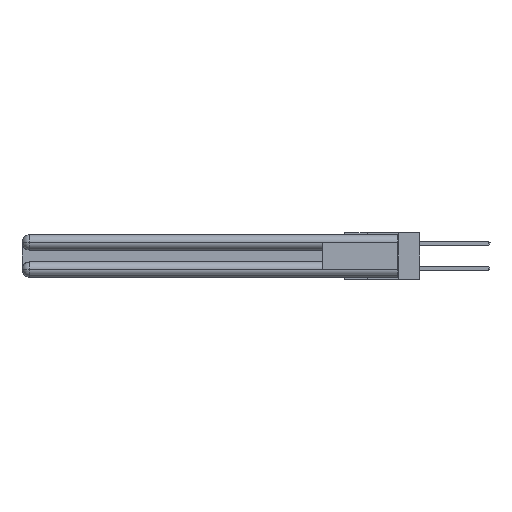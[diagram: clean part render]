
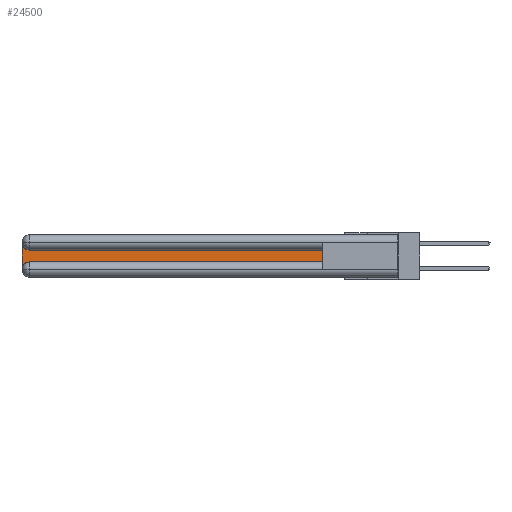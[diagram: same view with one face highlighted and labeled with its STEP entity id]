
A CAD part, left-side view. The second image highlights one B-rep face of the part: STEP entity #24500.
In plain terms, the highlighted planar face has unit normal (-1, 0, 0).
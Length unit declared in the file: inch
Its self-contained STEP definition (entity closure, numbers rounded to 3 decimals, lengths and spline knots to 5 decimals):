
#198 = DIRECTION ( 'NONE',  ( 0., 0., 1. ) ) ;
#234 = CARTESIAN_POINT ( 'NONE',  ( 0.075, 2.94, -0.0625 ) ) ;
#450 = ORIENTED_EDGE ( 'NONE', *, *, #9087, .T. ) ;
#917 = LINE ( 'NONE', #4924, #21539 ) ;
#2057 = VERTEX_POINT ( 'NONE', #13671 ) ;
#2864 = CARTESIAN_POINT ( 'NONE',  ( 0.075, 2.94, -0.2775 ) ) ;
#3566 = EDGE_CURVE ( 'NONE', #9020, #15563, #11306, .T. ) ;
#3692 = CARTESIAN_POINT ( 'NONE',  ( 0.075, 2.94, -0.1225 ) ) ;
#3745 = LINE ( 'NONE', #21882, #11422 ) ;
#3934 = DIRECTION ( 'NONE',  ( 0., 1., 0. ) ) ;
#4924 = CARTESIAN_POINT ( 'NONE',  ( 0.075, 0.6, -0.2175 ) ) ;
#5895 = ORIENTED_EDGE ( 'NONE', *, *, #7381, .T. ) ;
#5934 = CARTESIAN_POINT ( 'NONE',  ( 0.075, 3., -0.2175 ) ) ;
#6162 = DIRECTION ( 'NONE',  ( 0., 0., -1. ) ) ;
#6202 = ORIENTED_EDGE ( 'NONE', *, *, #17113, .T. ) ;
#6261 = VERTEX_POINT ( 'NONE', #22116 ) ;
#6617 = DIRECTION ( 'NONE',  ( 0., -1., 0. ) ) ;
#7381 = EDGE_CURVE ( 'NONE', #16504, #6261, #18787, .T. ) ;
#8151 = FACE_OUTER_BOUND ( 'NONE', #25121, .T. ) ;
#9020 = VERTEX_POINT ( 'NONE', #3692 ) ;
#9087 = EDGE_CURVE ( 'NONE', #6261, #12498, #3745, .T. ) ;
#10647 = PLANE ( 'NONE',  #30736 ) ;
#10774 = CARTESIAN_POINT ( 'NONE',  ( 0.075, 3., -0.2775 ) ) ;
#11306 = CIRCLE ( 'NONE', #14904, 0.06 ) ;
#11422 = VECTOR ( 'NONE', #6617, 39.37008 ) ;
#11513 = LINE ( 'NONE', #16531, #30463 ) ;
#12498 = VERTEX_POINT ( 'NONE', #12693 ) ;
#12693 = CARTESIAN_POINT ( 'NONE',  ( 0.075, 0.6, -0.2175 ) ) ;
#12757 = DIRECTION ( 'NONE',  ( 1., 0., 0. ) ) ;
#13257 = DIRECTION ( 'NONE',  ( 1., 0., 0. ) ) ;
#13493 = DIRECTION ( 'NONE',  ( 0., 0., -1. ) ) ;
#13644 = CARTESIAN_POINT ( 'NONE',  ( 0.075, 3., -0.0625 ) ) ;
#13671 = CARTESIAN_POINT ( 'NONE',  ( 0.075, 0.6, -0.1225 ) ) ;
#14376 = DIRECTION ( 'NONE',  ( 0., 0., -1. ) ) ;
#14653 = LINE ( 'NONE', #5934, #27131 ) ;
#14904 = AXIS2_PLACEMENT_3D ( 'NONE', #234, #13257, #13493 ) ;
#15563 = VERTEX_POINT ( 'NONE', #13644 ) ;
#15821 = DIRECTION ( 'NONE',  ( 0., 0., -1. ) ) ;
#16258 = EDGE_CURVE ( 'NONE', #12498, #2057, #917, .T. ) ;
#16504 = VERTEX_POINT ( 'NONE', #10774 ) ;
#16531 = CARTESIAN_POINT ( 'NONE',  ( 0.075, 0.6, -0.1225 ) ) ;
#17113 = EDGE_CURVE ( 'NONE', #15563, #16504, #14653, .T. ) ;
#18787 = CIRCLE ( 'NONE', #24936, 0.06 ) ;
#21539 = VECTOR ( 'NONE', #198, 39.37008 ) ;
#21659 = ORIENTED_EDGE ( 'NONE', *, *, #16258, .T. ) ;
#21882 = CARTESIAN_POINT ( 'NONE',  ( 0.075, 0.6, -0.2175 ) ) ;
#22116 = CARTESIAN_POINT ( 'NONE',  ( 0.075, 2.94, -0.2175 ) ) ;
#23326 = EDGE_CURVE ( 'NONE', #2057, #9020, #11513, .T. ) ;
#23646 = CARTESIAN_POINT ( 'NONE',  ( 0.075, 3., -0.1225 ) ) ;
#24500 = ADVANCED_FACE ( 'NONE', ( #8151 ), #10647, .F. ) ;
#24936 = AXIS2_PLACEMENT_3D ( 'NONE', #2864, #12757, #15821 ) ;
#25121 = EDGE_LOOP ( 'NONE', ( #29835, #25685, #6202, #5895, #450, #21659 ) ) ;
#25685 = ORIENTED_EDGE ( 'NONE', *, *, #3566, .T. ) ;
#26251 = DIRECTION ( 'NONE',  ( 1., 0., 0. ) ) ;
#27131 = VECTOR ( 'NONE', #6162, 39.37008 ) ;
#29835 = ORIENTED_EDGE ( 'NONE', *, *, #23326, .T. ) ;
#30463 = VECTOR ( 'NONE', #3934, 39.37008 ) ;
#30736 = AXIS2_PLACEMENT_3D ( 'NONE', #23646, #26251, #14376 ) ;
